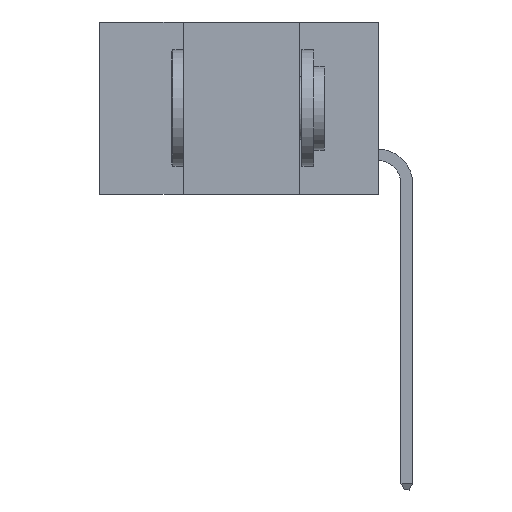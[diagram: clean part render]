
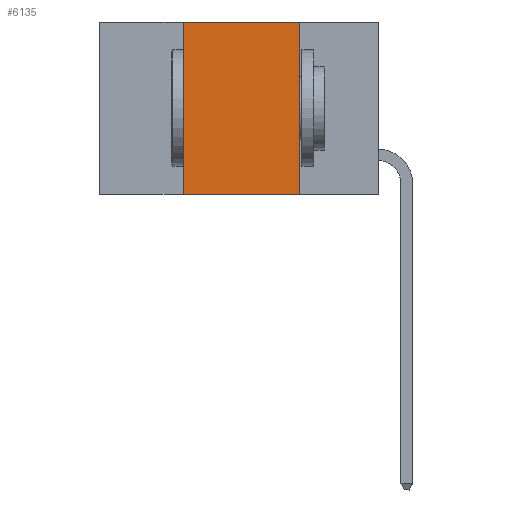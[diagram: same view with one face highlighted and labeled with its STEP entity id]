
A CAD part, left-side view. The second image highlights one B-rep face of the part: STEP entity #6135.
In plain terms, the highlighted planar face has unit normal (-1, 0, 0).
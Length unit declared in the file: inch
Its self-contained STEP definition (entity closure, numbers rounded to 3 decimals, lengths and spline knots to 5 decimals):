
#29 = DIRECTION ( 'NONE',  ( 0., 0., -1. ) ) ;
#49 = VECTOR ( 'NONE', #9507, 39.37008 ) ;
#869 = VECTOR ( 'NONE', #2596, 39.37008 ) ;
#902 = VECTOR ( 'NONE', #5797, 39.37008 ) ;
#1299 = DIRECTION ( 'NONE',  ( 1., 0., 0. ) ) ;
#2262 = ORIENTED_EDGE ( 'NONE', *, *, #8390, .F. ) ;
#2429 = LINE ( 'NONE', #10919, #869 ) ;
#2480 = VERTEX_POINT ( 'NONE', #6147 ) ;
#2596 = DIRECTION ( 'NONE',  ( 0., -1., 0. ) ) ;
#2950 = DIRECTION ( 'NONE',  ( 0., 0., -1. ) ) ;
#3570 = EDGE_LOOP ( 'NONE', ( #10690, #2262, #6888, #5526 ) ) ;
#4060 = FACE_OUTER_BOUND ( 'NONE', #3570, .T. ) ;
#4824 = CARTESIAN_POINT ( 'NONE',  ( 0., 0.6, 0. ) ) ;
#5526 = ORIENTED_EDGE ( 'NONE', *, *, #9418, .T. ) ;
#5537 = CARTESIAN_POINT ( 'NONE',  ( 0., 0.17, -0.37 ) ) ;
#5724 = LINE ( 'NONE', #7278, #10442 ) ;
#5797 = DIRECTION ( 'NONE',  ( 0., -1., 0. ) ) ;
#6039 = LINE ( 'NONE', #11279, #902 ) ;
#6135 = ADVANCED_FACE ( 'NONE', ( #4060 ), #10302, .F. ) ;
#6141 = AXIS2_PLACEMENT_3D ( 'NONE', #4824, #1299, #2950 ) ;
#6147 = CARTESIAN_POINT ( 'NONE',  ( 0., 0.17, 0. ) ) ;
#6445 = LINE ( 'NONE', #7742, #49 ) ;
#6888 = ORIENTED_EDGE ( 'NONE', *, *, #8326, .F. ) ;
#7278 = CARTESIAN_POINT ( 'NONE',  ( 0., 0.17, 0. ) ) ;
#7456 = VERTEX_POINT ( 'NONE', #5537 ) ;
#7464 = CARTESIAN_POINT ( 'NONE',  ( 0., 0.42, 0. ) ) ;
#7742 = CARTESIAN_POINT ( 'NONE',  ( 0., 0.42, 0. ) ) ;
#8326 = EDGE_CURVE ( 'NONE', #9622, #11803, #6445, .T. ) ;
#8390 = EDGE_CURVE ( 'NONE', #11803, #2480, #6039, .T. ) ;
#9015 = EDGE_CURVE ( 'NONE', #2480, #7456, #5724, .T. ) ;
#9418 = EDGE_CURVE ( 'NONE', #9622, #7456, #2429, .T. ) ;
#9507 = DIRECTION ( 'NONE',  ( 0., 0., 1. ) ) ;
#9622 = VERTEX_POINT ( 'NONE', #10495 ) ;
#10302 = PLANE ( 'NONE',  #6141 ) ;
#10442 = VECTOR ( 'NONE', #29, 39.37008 ) ;
#10495 = CARTESIAN_POINT ( 'NONE',  ( 0., 0.42, -0.37 ) ) ;
#10690 = ORIENTED_EDGE ( 'NONE', *, *, #9015, .F. ) ;
#10919 = CARTESIAN_POINT ( 'NONE',  ( 0., 0.6, -0.37 ) ) ;
#11279 = CARTESIAN_POINT ( 'NONE',  ( 0., 0.6, 0. ) ) ;
#11803 = VERTEX_POINT ( 'NONE', #7464 ) ;
